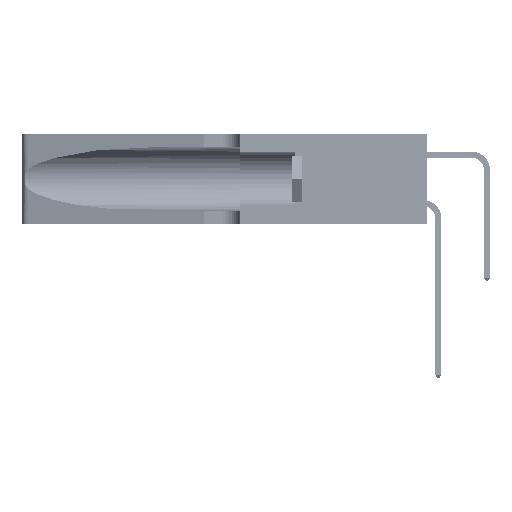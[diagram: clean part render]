
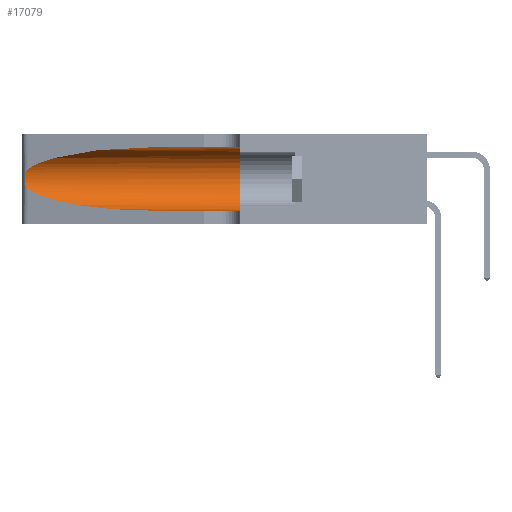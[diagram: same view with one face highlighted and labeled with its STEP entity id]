
A CAD part, left-side view. The second image highlights one B-rep face of the part: STEP entity #17079.
In plain terms, the highlighted cylindrical face has radius 3.308 mm (diameter 6.617 mm), a partial arc.
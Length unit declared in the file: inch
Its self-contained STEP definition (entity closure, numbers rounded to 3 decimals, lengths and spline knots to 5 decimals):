
#258 = CARTESIAN_POINT ( 'NONE',  ( 0.25487, 1.22718, 0.22369 ) ) ;
#1123 = CARTESIAN_POINT ( 'NONE',  ( 0.1305, 0.72297, 0.31525 ) ) ;
#1418 = CARTESIAN_POINT ( 'NONE',  ( 0.25639, 1.23184, 0.21858 ) ) ;
#1597 = CARTESIAN_POINT ( 'NONE',  ( 0.25856, 1.23593, 0.16098 ) ) ;
#2631 = ORIENTED_EDGE ( 'NONE', *, *, #49683, .F. ) ;
#4370 = ORIENTED_EDGE ( 'NONE', *, *, #8830, .T. ) ;
#4715 = AXIS2_PLACEMENT_3D ( 'NONE', #23805, #27795, #43265 ) ;
#5207 = CARTESIAN_POINT ( 'NONE',  ( 0.18966, 0.96281, 0.31525 ) ) ;
#5508 = CARTESIAN_POINT ( 'NONE',  ( 0.25555, 1.22994, 0.2215 ) ) ;
#5672 = CARTESIAN_POINT ( 'NONE',  ( 0.25639, 1.23186, 0.15144 ) ) ;
#5943 = CARTESIAN_POINT ( 'NONE',  ( 0.1305, 1.61858, 0.05475 ) ) ;
#6391 = EDGE_CURVE ( 'NONE', #13941, #18684, #49050, .T. ) ;
#6476 = DIRECTION ( 'NONE',  ( 0., 1., 0. ) ) ;
#6645 = CARTESIAN_POINT ( 'NONE',  ( 0.2373, 1.15595, 0.08982 ) ) ;
#8830 = EDGE_CURVE ( 'NONE', #28424, #10078, #19128, .T. ) ;
#9207 = CARTESIAN_POINT ( 'NONE',  ( 0.25487, 1.22718, 0.22369 ) ) ;
#9399 = EDGE_CURVE ( 'NONE', #50248, #13941, #50636, .T. ) ;
#9670 = CARTESIAN_POINT ( 'NONE',  ( 0.25487, 1.22718, 0.14631 ) ) ;
#10078 = VERTEX_POINT ( 'NONE', #48427 ) ;
#10212 =( BOUNDED_CURVE ( )  B_SPLINE_CURVE ( 3, ( #26377, #6645, #38227, #14618 ),
 .UNSPECIFIED., .F., .F. ) 
 B_SPLINE_CURVE_WITH_KNOTS ( ( 4, 4 ),
 ( 3.44316, 4.71239 ),
 .UNSPECIFIED. ) 
 CURVE ( )  GEOMETRIC_REPRESENTATION_ITEM ( )  RATIONAL_B_SPLINE_CURVE ( ( 1., 0.87, 0.87, 1. ) ) 
 REPRESENTATION_ITEM ( '' )  );
#13480 = CARTESIAN_POINT ( 'NONE',  ( 0.25487, 1.22718, 0.22369 ) ) ;
#13598 = DIRECTION ( 'NONE',  ( 0., -1., 0. ) ) ;
#13941 = VERTEX_POINT ( 'NONE', #258 ) ;
#14582 = CARTESIAN_POINT ( 'NONE',  ( 0.1305, 0.72297, 0.31525 ) ) ;
#14618 = CARTESIAN_POINT ( 'NONE',  ( 0.1305, 0.72297, 0.05475 ) ) ;
#17079 = ADVANCED_FACE ( 'NONE', ( #42035 ), #19889, .F. ) ;
#17489 = CARTESIAN_POINT ( 'NONE',  ( 0.25854, 1.2359, 0.20912 ) ) ;
#18026 = CARTESIAN_POINT ( 'NONE',  ( 0.1305, 1.61858, 0.31525 ) ) ;
#18684 = VERTEX_POINT ( 'NONE', #33472 ) ;
#19128 = LINE ( 'NONE', #5943, #38814 ) ;
#19273 = ORIENTED_EDGE ( 'NONE', *, *, #41361, .T. ) ;
#19889 = CYLINDRICAL_SURFACE ( 'NONE', #4715, 0.13025 ) ;
#21450 = CARTESIAN_POINT ( 'NONE',  ( 0.26075, 1.23896, 0.19203 ) ) ;
#23805 = CARTESIAN_POINT ( 'NONE',  ( 0.1305, 1.61858, 0.185 ) ) ;
#24701 = CARTESIAN_POINT ( 'NONE',  ( 0.1305, 0.72297, 0.05475 ) ) ;
#24802 = EDGE_CURVE ( 'NONE', #50248, #39912, #33191, .T. ) ;
#25396 = CARTESIAN_POINT ( 'NONE',  ( 0.26017, 1.23833, 0.17102 ) ) ;
#25736 = ORIENTED_EDGE ( 'NONE', *, *, #6391, .T. ) ;
#26377 = CARTESIAN_POINT ( 'NONE',  ( 0.25487, 1.22718, 0.14631 ) ) ;
#27795 = DIRECTION ( 'NONE',  ( 0., -1., 0. ) ) ;
#28424 = VERTEX_POINT ( 'NONE', #24701 ) ;
#29086 = CARTESIAN_POINT ( 'NONE',  ( 0.1305, 0.35, 0.31525 ) ) ;
#29362 = CARTESIAN_POINT ( 'NONE',  ( 0.25789, 1.23486, 0.15765 ) ) ;
#30058 = ORIENTED_EDGE ( 'NONE', *, *, #9399, .T. ) ;
#30150 = CARTESIAN_POINT ( 'NONE',  ( 0.1305, 0.35, 0.185 ) ) ;
#30517 = AXIS2_PLACEMENT_3D ( 'NONE', #30150, #6476, #34084 ) ;
#32844 = CARTESIAN_POINT ( 'NONE',  ( 0.2373, 1.15595, 0.28018 ) ) ;
#33191 = LINE ( 'NONE', #18026, #43644 ) ;
#33304 = CARTESIAN_POINT ( 'NONE',  ( 0.25555, 1.22993, 0.14849 ) ) ;
#33472 = CARTESIAN_POINT ( 'NONE',  ( 0.25487, 1.22718, 0.14631 ) ) ;
#34084 = DIRECTION ( 'NONE',  ( 0., 0., 1. ) ) ;
#37630 = DIRECTION ( 'NONE',  ( 0., -1., 0. ) ) ;
#38227 = CARTESIAN_POINT ( 'NONE',  ( 0.18966, 0.96281, 0.05475 ) ) ;
#38814 = VECTOR ( 'NONE', #13598, 39.37008 ) ;
#39912 = VERTEX_POINT ( 'NONE', #29086 ) ;
#41051 = CARTESIAN_POINT ( 'NONE',  ( 0.25787, 1.23484, 0.2124 ) ) ;
#41361 = EDGE_CURVE ( 'NONE', #18684, #28424, #10212, .T. ) ;
#42035 = FACE_OUTER_BOUND ( 'NONE', #50231, .T. ) ;
#43265 = DIRECTION ( 'NONE',  ( 0., 0., -1. ) ) ;
#43644 = VECTOR ( 'NONE', #37630, 39.37008 ) ;
#44703 = ORIENTED_EDGE ( 'NONE', *, *, #24802, .F. ) ;
#44996 = CARTESIAN_POINT ( 'NONE',  ( 0.26018, 1.23835, 0.19895 ) ) ;
#46753 = CIRCLE ( 'NONE', #30517, 0.13025 ) ;
#48427 = CARTESIAN_POINT ( 'NONE',  ( 0.1305, 0.35, 0.05475 ) ) ;
#48935 = CARTESIAN_POINT ( 'NONE',  ( 0.26075, 1.23896, 0.178 ) ) ;
#49050 = B_SPLINE_CURVE_WITH_KNOTS ( 'NONE', 3,
 ( #13480, #5508, #1418, #41051, #17489, #44996, #21450, #48935, #25396, #1597, #29362, #5672, #33304, #9670 ),
 .UNSPECIFIED., .F., .F.,
 ( 4, 2, 2, 2, 2, 2, 4 ),
 ( 0., 0.00027, 0.00053, 0.00107, 0.0016, 0.00187, 0.00214 ),
 .UNSPECIFIED. ) ;
#49683 = EDGE_CURVE ( 'NONE', #39912, #10078, #46753, .T. ) ;
#50231 = EDGE_LOOP ( 'NONE', ( #30058, #25736, #19273, #4370, #2631, #44703 ) ) ;
#50248 = VERTEX_POINT ( 'NONE', #14582 ) ;
#50636 =( BOUNDED_CURVE ( )  B_SPLINE_CURVE ( 3, ( #1123, #5207, #32844, #9207 ),
 .UNSPECIFIED., .F., .T. ) 
 B_SPLINE_CURVE_WITH_KNOTS ( ( 4, 4 ),
 ( 1.5708, 2.84003 ),
 .UNSPECIFIED. ) 
 CURVE ( )  GEOMETRIC_REPRESENTATION_ITEM ( )  RATIONAL_B_SPLINE_CURVE ( ( 1., 0.87, 0.87, 1. ) ) 
 REPRESENTATION_ITEM ( '' )  );
